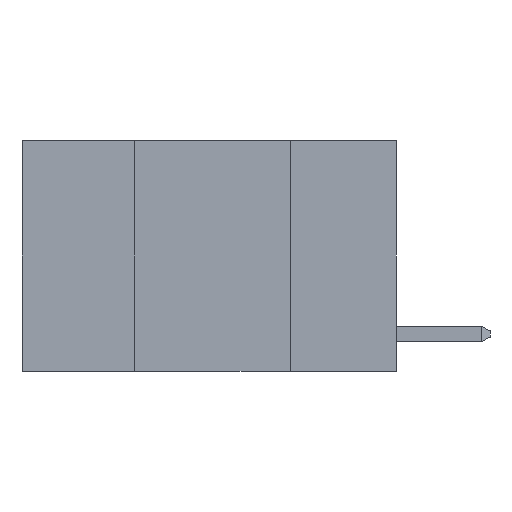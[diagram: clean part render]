
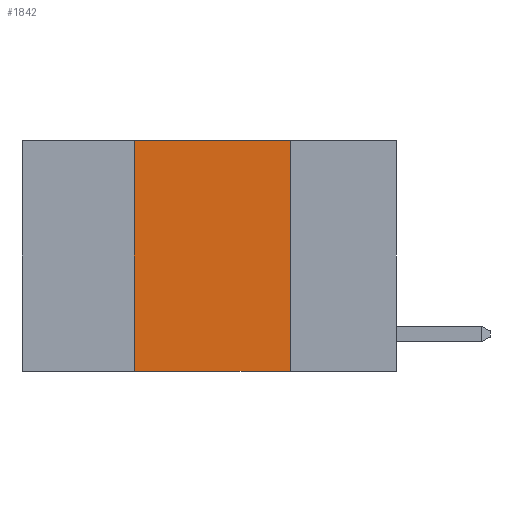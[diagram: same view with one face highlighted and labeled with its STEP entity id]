
A CAD part, left-side view. The second image highlights one B-rep face of the part: STEP entity #1842.
In plain terms, the highlighted planar face has unit normal (-1, 0, 0).
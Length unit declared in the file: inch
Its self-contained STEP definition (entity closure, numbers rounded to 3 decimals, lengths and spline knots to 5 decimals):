
#331 = ORIENTED_EDGE ( 'NONE', *, *, #6871, .F. ) ;
#338 = DIRECTION ( 'NONE',  ( 0., 0., 1. ) ) ;
#1807 = LINE ( 'NONE', #6052, #5737 ) ;
#1827 = ORIENTED_EDGE ( 'NONE', *, *, #4794, .T. ) ;
#1842 = ADVANCED_FACE ( 'NONE', ( #7426 ), #3210, .F. ) ;
#1960 = EDGE_CURVE ( 'NONE', #7968, #9060, #4679, .T. ) ;
#2131 = DIRECTION ( 'NONE',  ( 0., -1., 0. ) ) ;
#2633 = CARTESIAN_POINT ( 'NONE',  ( 0., 0.6, 0. ) ) ;
#2915 = ORIENTED_EDGE ( 'NONE', *, *, #1960, .F. ) ;
#3131 = DIRECTION ( 'NONE',  ( 0., 0., -1. ) ) ;
#3132 = ORIENTED_EDGE ( 'NONE', *, *, #4784, .F. ) ;
#3181 = CARTESIAN_POINT ( 'NONE',  ( 0., 0.6, 0. ) ) ;
#3210 = PLANE ( 'NONE',  #8458 ) ;
#3271 = DIRECTION ( 'NONE',  ( 1., 0., 0. ) ) ;
#3283 = LINE ( 'NONE', #2633, #8937 ) ;
#4172 = VECTOR ( 'NONE', #8715, 39.37008 ) ;
#4204 = CARTESIAN_POINT ( 'NONE',  ( 0., 0.42, 0. ) ) ;
#4679 = LINE ( 'NONE', #8159, #4172 ) ;
#4784 = EDGE_CURVE ( 'NONE', #9654, #5653, #10176, .T. ) ;
#4794 = EDGE_CURVE ( 'NONE', #9654, #9060, #1807, .T. ) ;
#5437 = CARTESIAN_POINT ( 'NONE',  ( 0., 0.17, 0. ) ) ;
#5653 = VERTEX_POINT ( 'NONE', #4204 ) ;
#5737 = VECTOR ( 'NONE', #2131, 39.37008 ) ;
#6016 = CARTESIAN_POINT ( 'NONE',  ( 0., 0.42, 0. ) ) ;
#6052 = CARTESIAN_POINT ( 'NONE',  ( 0., 0.6, -0.37 ) ) ;
#6217 = CARTESIAN_POINT ( 'NONE',  ( 0., 0.42, -0.37 ) ) ;
#6494 = CARTESIAN_POINT ( 'NONE',  ( 0., 0.17, -0.37 ) ) ;
#6544 = DIRECTION ( 'NONE',  ( 0., -1., 0. ) ) ;
#6871 = EDGE_CURVE ( 'NONE', #5653, #7968, #3283, .T. ) ;
#7426 = FACE_OUTER_BOUND ( 'NONE', #8267, .T. ) ;
#7968 = VERTEX_POINT ( 'NONE', #5437 ) ;
#8004 = VECTOR ( 'NONE', #338, 39.37008 ) ;
#8159 = CARTESIAN_POINT ( 'NONE',  ( 0., 0.17, 0. ) ) ;
#8267 = EDGE_LOOP ( 'NONE', ( #2915, #331, #3132, #1827 ) ) ;
#8458 = AXIS2_PLACEMENT_3D ( 'NONE', #3181, #3271, #3131 ) ;
#8715 = DIRECTION ( 'NONE',  ( 0., 0., -1. ) ) ;
#8937 = VECTOR ( 'NONE', #6544, 39.37008 ) ;
#9060 = VERTEX_POINT ( 'NONE', #6494 ) ;
#9654 = VERTEX_POINT ( 'NONE', #6217 ) ;
#10176 = LINE ( 'NONE', #6016, #8004 ) ;
